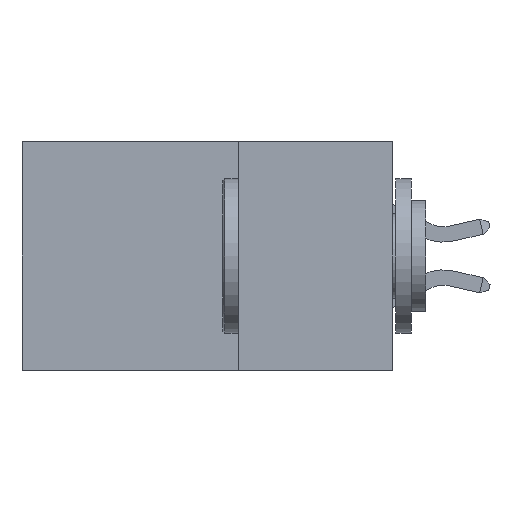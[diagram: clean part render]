
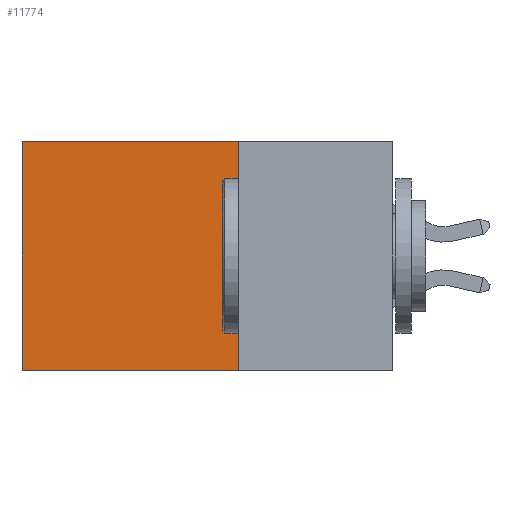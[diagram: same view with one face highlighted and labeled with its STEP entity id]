
A CAD part, left-side view. The second image highlights one B-rep face of the part: STEP entity #11774.
In plain terms, the highlighted planar face has unit normal (-1, 0, 0).
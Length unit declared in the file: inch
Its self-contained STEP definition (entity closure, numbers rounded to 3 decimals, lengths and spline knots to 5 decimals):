
#621 = CARTESIAN_POINT ( 'NONE',  ( 0.2875, 0.25, 0. ) ) ;
#1240 = DIRECTION ( 'NONE',  ( 0., 0., -1. ) ) ;
#2231 = CARTESIAN_POINT ( 'NONE',  ( 0.2875, 0.6, 0. ) ) ;
#2386 = ORIENTED_EDGE ( 'NONE', *, *, #10983, .T. ) ;
#2880 = CARTESIAN_POINT ( 'NONE',  ( 0.2875, 0.6, -0.37 ) ) ;
#3267 = LINE ( 'NONE', #12841, #6910 ) ;
#4420 = DIRECTION ( 'NONE',  ( 0., 0., -1. ) ) ;
#4450 = LINE ( 'NONE', #621, #9536 ) ;
#4650 = ORIENTED_EDGE ( 'NONE', *, *, #6918, .F. ) ;
#5000 = CARTESIAN_POINT ( 'NONE',  ( 0.2875, 0.25, 0. ) ) ;
#5638 = EDGE_CURVE ( 'NONE', #10372, #5656, #16504, .T. ) ;
#5656 = VERTEX_POINT ( 'NONE', #2880 ) ;
#6106 = ORIENTED_EDGE ( 'NONE', *, *, #8830, .F. ) ;
#6904 = FACE_OUTER_BOUND ( 'NONE', #13932, .T. ) ;
#6910 = VECTOR ( 'NONE', #10509, 39.37008 ) ;
#6918 = EDGE_CURVE ( 'NONE', #12044, #5656, #3267, .T. ) ;
#7519 = VERTEX_POINT ( 'NONE', #5000 ) ;
#7735 = VECTOR ( 'NONE', #4420, 39.37008 ) ;
#7972 = PLANE ( 'NONE',  #12449 ) ;
#8830 = EDGE_CURVE ( 'NONE', #7519, #12044, #15381, .T. ) ;
#9443 = CARTESIAN_POINT ( 'NONE',  ( 0.2875, 0.25, 0. ) ) ;
#9536 = VECTOR ( 'NONE', #14225, 39.37008 ) ;
#9541 = ORIENTED_EDGE ( 'NONE', *, *, #5638, .T. ) ;
#10372 = VERTEX_POINT ( 'NONE', #12656 ) ;
#10509 = DIRECTION ( 'NONE',  ( 0., 1., 0. ) ) ;
#10846 = DIRECTION ( 'NONE',  ( 1., 0., 0. ) ) ;
#10983 = EDGE_CURVE ( 'NONE', #7519, #10372, #4450, .T. ) ;
#10997 = CARTESIAN_POINT ( 'NONE',  ( 0.2875, 0.25, -0.37 ) ) ;
#11267 = CARTESIAN_POINT ( 'NONE',  ( 0.2875, 0.25, 0. ) ) ;
#11774 = ADVANCED_FACE ( 'NONE', ( #6904 ), #7972, .F. ) ;
#12044 = VERTEX_POINT ( 'NONE', #10997 ) ;
#12449 = AXIS2_PLACEMENT_3D ( 'NONE', #9443, #10846, #1240 ) ;
#12656 = CARTESIAN_POINT ( 'NONE',  ( 0.2875, 0.6, 0. ) ) ;
#12841 = CARTESIAN_POINT ( 'NONE',  ( 0.2875, 0.25, -0.37 ) ) ;
#13932 = EDGE_LOOP ( 'NONE', ( #9541, #4650, #6106, #2386 ) ) ;
#14225 = DIRECTION ( 'NONE',  ( 0., 1., 0. ) ) ;
#15381 = LINE ( 'NONE', #11267, #7735 ) ;
#16504 = LINE ( 'NONE', #2231, #17346 ) ;
#17263 = DIRECTION ( 'NONE',  ( 0., 0., -1. ) ) ;
#17346 = VECTOR ( 'NONE', #17263, 39.37008 ) ;
